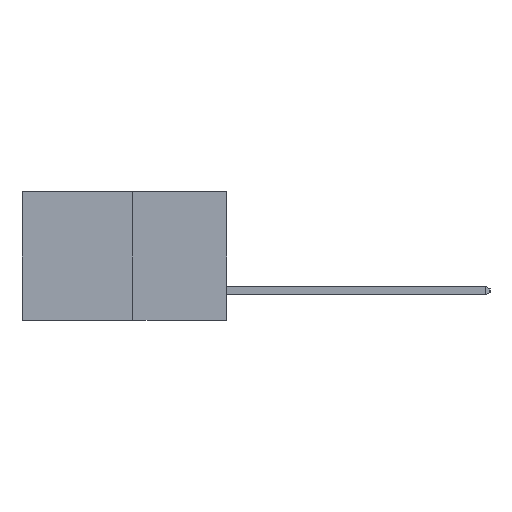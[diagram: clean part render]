
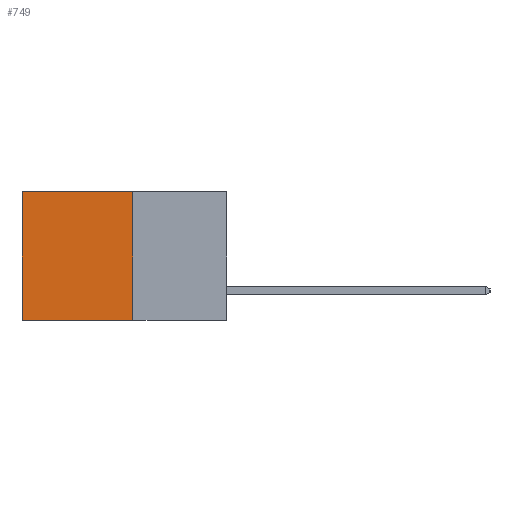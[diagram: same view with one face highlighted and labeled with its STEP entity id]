
A CAD part, left-side view. The second image highlights one B-rep face of the part: STEP entity #749.
In plain terms, the highlighted planar face has unit normal (-1, 0, 0).
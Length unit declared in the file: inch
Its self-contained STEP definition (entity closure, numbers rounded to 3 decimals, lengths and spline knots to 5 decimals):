
#470 = CARTESIAN_POINT ( 'NONE',  ( 0.277, 0.27, -0.37 ) ) ;
#650 = CARTESIAN_POINT ( 'NONE',  ( 0.277, 0.27, 0. ) ) ;
#749 = ADVANCED_FACE ( 'NONE', ( #9225 ), #14448, .F. ) ;
#1669 = EDGE_CURVE ( 'NONE', #7190, #4250, #11742, .T. ) ;
#2087 = ORIENTED_EDGE ( 'NONE', *, *, #5385, .F. ) ;
#2436 = CARTESIAN_POINT ( 'NONE',  ( 0.277, 0.59, 0. ) ) ;
#2518 = EDGE_CURVE ( 'NONE', #6037, #4250, #10234, .T. ) ;
#2838 = ORIENTED_EDGE ( 'NONE', *, *, #9986, .T. ) ;
#3289 = CARTESIAN_POINT ( 'NONE',  ( 0.277, 0.27, -0.37 ) ) ;
#3443 = DIRECTION ( 'NONE',  ( 1., 0., 0. ) ) ;
#4250 = VERTEX_POINT ( 'NONE', #8539 ) ;
#4331 = VECTOR ( 'NONE', #7192, 39.37008 ) ;
#4804 = CARTESIAN_POINT ( 'NONE',  ( 0.277, 0.59, -0.37 ) ) ;
#4869 = CARTESIAN_POINT ( 'NONE',  ( 0.277, 0.27, -0.37 ) ) ;
#5385 = EDGE_CURVE ( 'NONE', #9040, #7190, #8553, .T. ) ;
#5985 = VECTOR ( 'NONE', #11235, 39.37008 ) ;
#6037 = VERTEX_POINT ( 'NONE', #2436 ) ;
#7190 = VERTEX_POINT ( 'NONE', #10476 ) ;
#7192 = DIRECTION ( 'NONE',  ( 0., 0., -1. ) ) ;
#7325 = ORIENTED_EDGE ( 'NONE', *, *, #2518, .T. ) ;
#8228 = EDGE_LOOP ( 'NONE', ( #7325, #13567, #2087, #2838 ) ) ;
#8539 = CARTESIAN_POINT ( 'NONE',  ( 0.277, 0.59, -0.37 ) ) ;
#8553 = LINE ( 'NONE', #470, #5985 ) ;
#8840 = VECTOR ( 'NONE', #14454, 39.37008 ) ;
#9040 = VERTEX_POINT ( 'NONE', #14314 ) ;
#9225 = FACE_OUTER_BOUND ( 'NONE', #8228, .T. ) ;
#9485 = LINE ( 'NONE', #650, #12345 ) ;
#9986 = EDGE_CURVE ( 'NONE', #9040, #6037, #9485, .T. ) ;
#10234 = LINE ( 'NONE', #4804, #4331 ) ;
#10476 = CARTESIAN_POINT ( 'NONE',  ( 0.277, 0.27, -0.37 ) ) ;
#11235 = DIRECTION ( 'NONE',  ( 0., 0., -1. ) ) ;
#11386 = DIRECTION ( 'NONE',  ( 0., 0., -1. ) ) ;
#11420 = AXIS2_PLACEMENT_3D ( 'NONE', #3289, #3443, #11386 ) ;
#11742 = LINE ( 'NONE', #4869, #8840 ) ;
#12345 = VECTOR ( 'NONE', #13635, 39.37008 ) ;
#13567 = ORIENTED_EDGE ( 'NONE', *, *, #1669, .F. ) ;
#13635 = DIRECTION ( 'NONE',  ( 0., 1., 0. ) ) ;
#14314 = CARTESIAN_POINT ( 'NONE',  ( 0.277, 0.27, 0. ) ) ;
#14448 = PLANE ( 'NONE',  #11420 ) ;
#14454 = DIRECTION ( 'NONE',  ( 0., 1., 0. ) ) ;
